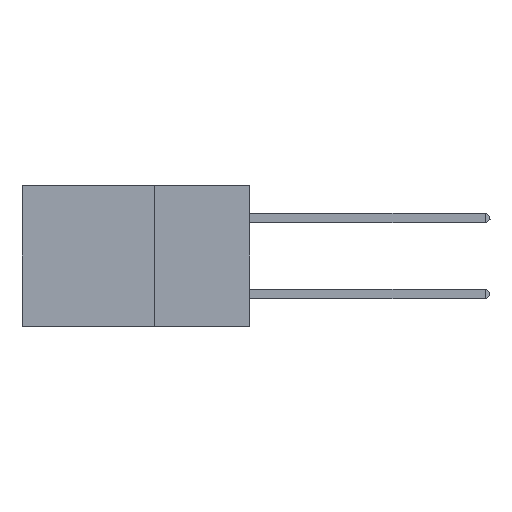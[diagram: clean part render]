
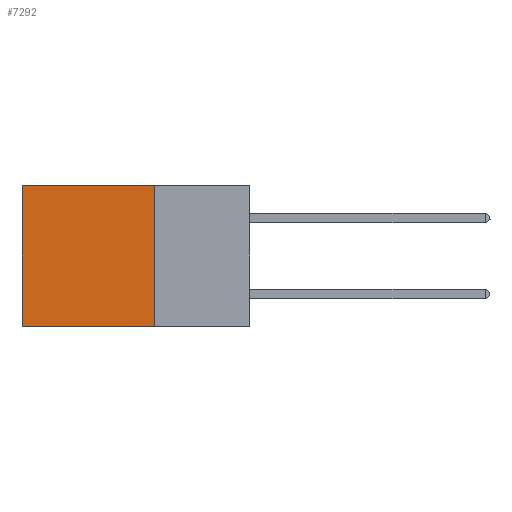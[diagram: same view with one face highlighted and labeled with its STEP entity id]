
A CAD part, left-side view. The second image highlights one B-rep face of the part: STEP entity #7292.
In plain terms, the highlighted planar face has unit normal (-1, 0, 0).
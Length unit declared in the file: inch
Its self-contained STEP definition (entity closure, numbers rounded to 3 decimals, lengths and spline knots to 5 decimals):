
#1016 = DIRECTION ( 'NONE',  ( 0., 0., -1. ) ) ;
#2571 = CARTESIAN_POINT ( 'NONE',  ( 0.2875, 0.25, 0. ) ) ;
#3425 = ORIENTED_EDGE ( 'NONE', *, *, #12012, .T. ) ;
#4088 = CARTESIAN_POINT ( 'NONE',  ( 0.2875, 0.25, 0. ) ) ;
#4135 = VERTEX_POINT ( 'NONE', #9559 ) ;
#4163 = ORIENTED_EDGE ( 'NONE', *, *, #5658, .F. ) ;
#4492 = FACE_OUTER_BOUND ( 'NONE', #11634, .T. ) ;
#4712 = CARTESIAN_POINT ( 'NONE',  ( 0.2875, 0.6, -0.37 ) ) ;
#5148 = CARTESIAN_POINT ( 'NONE',  ( 0.2875, 0.25, -0.37 ) ) ;
#5658 = EDGE_CURVE ( 'NONE', #17643, #4135, #23689, .T. ) ;
#6332 = AXIS2_PLACEMENT_3D ( 'NONE', #15651, #19833, #1016 ) ;
#6557 = EDGE_CURVE ( 'NONE', #4135, #12005, #7477, .T. ) ;
#6639 = VERTEX_POINT ( 'NONE', #21114 ) ;
#6787 = LINE ( 'NONE', #10102, #21356 ) ;
#7242 = ORIENTED_EDGE ( 'NONE', *, *, #6557, .F. ) ;
#7292 = ADVANCED_FACE ( 'NONE', ( #4492 ), #17489, .F. ) ;
#7477 = LINE ( 'NONE', #5148, #23187 ) ;
#9559 = CARTESIAN_POINT ( 'NONE',  ( 0.2875, 0.25, -0.37 ) ) ;
#9861 = LINE ( 'NONE', #4088, #11305 ) ;
#10102 = CARTESIAN_POINT ( 'NONE',  ( 0.2875, 0.6, 0. ) ) ;
#11305 = VECTOR ( 'NONE', #19079, 39.37008 ) ;
#11634 = EDGE_LOOP ( 'NONE', ( #3425, #7242, #4163, #15059 ) ) ;
#12005 = VERTEX_POINT ( 'NONE', #4712 ) ;
#12012 = EDGE_CURVE ( 'NONE', #6639, #12005, #6787, .T. ) ;
#15059 = ORIENTED_EDGE ( 'NONE', *, *, #23156, .T. ) ;
#15651 = CARTESIAN_POINT ( 'NONE',  ( 0.2875, 0.25, 0. ) ) ;
#17489 = PLANE ( 'NONE',  #6332 ) ;
#17643 = VERTEX_POINT ( 'NONE', #2571 ) ;
#17833 = DIRECTION ( 'NONE',  ( 0., 0., -1. ) ) ;
#17993 = DIRECTION ( 'NONE',  ( 0., 0., -1. ) ) ;
#19079 = DIRECTION ( 'NONE',  ( 0., 1., 0. ) ) ;
#19833 = DIRECTION ( 'NONE',  ( 1., 0., 0. ) ) ;
#21114 = CARTESIAN_POINT ( 'NONE',  ( 0.2875, 0.6, 0. ) ) ;
#21356 = VECTOR ( 'NONE', #17833, 39.37008 ) ;
#22115 = DIRECTION ( 'NONE',  ( 0., 1., 0. ) ) ;
#22336 = CARTESIAN_POINT ( 'NONE',  ( 0.2875, 0.25, 0. ) ) ;
#22777 = VECTOR ( 'NONE', #17993, 39.37008 ) ;
#23156 = EDGE_CURVE ( 'NONE', #17643, #6639, #9861, .T. ) ;
#23187 = VECTOR ( 'NONE', #22115, 39.37008 ) ;
#23689 = LINE ( 'NONE', #22336, #22777 ) ;
